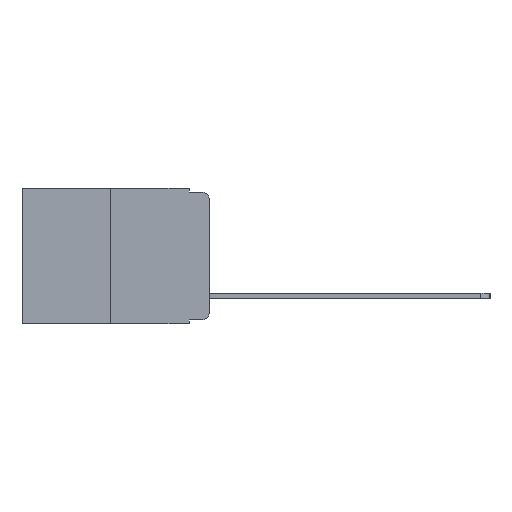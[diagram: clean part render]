
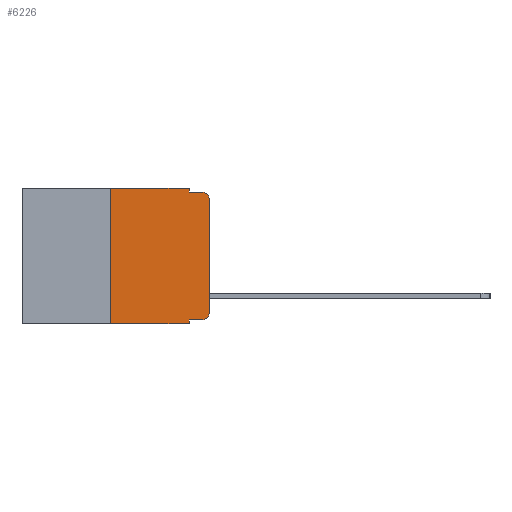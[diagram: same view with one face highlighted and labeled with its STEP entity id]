
A CAD part, left-side view. The second image highlights one B-rep face of the part: STEP entity #6226.
In plain terms, the highlighted planar face has unit normal (-1, 0, 0).
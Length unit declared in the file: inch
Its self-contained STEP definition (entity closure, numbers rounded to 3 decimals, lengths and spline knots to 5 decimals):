
#80 = DIRECTION ( 'NONE',  ( 0., -1., 0. ) ) ;
#190 = CARTESIAN_POINT ( 'NONE',  ( 0., 0.473, 0. ) ) ;
#302 = VERTEX_POINT ( 'NONE', #14236 ) ;
#464 = LINE ( 'NONE', #7982, #3529 ) ;
#611 = VERTEX_POINT ( 'NONE', #10614 ) ;
#622 = ORIENTED_EDGE ( 'NONE', *, *, #9368, .F. ) ;
#929 = EDGE_CURVE ( 'NONE', #302, #2626, #15216, .T. ) ;
#1022 = DIRECTION ( 'NONE',  ( -1., 0., 0. ) ) ;
#1023 = DIRECTION ( 'NONE',  ( 0., 0., -1. ) ) ;
#1599 = DIRECTION ( 'NONE',  ( 1., 0., 0. ) ) ;
#1757 = EDGE_CURVE ( 'NONE', #7967, #7173, #464, .T. ) ;
#2019 = CARTESIAN_POINT ( 'NONE',  ( 0., 0.25, 0. ) ) ;
#2097 = VECTOR ( 'NONE', #10262, 39.37008 ) ;
#2626 = VERTEX_POINT ( 'NONE', #9595 ) ;
#2838 = PLANE ( 'NONE',  #9090 ) ;
#2847 = ORIENTED_EDGE ( 'NONE', *, *, #3936, .F. ) ;
#2858 = LINE ( 'NONE', #5931, #15145 ) ;
#2879 = EDGE_CURVE ( 'NONE', #7972, #7967, #13456, .T. ) ;
#2944 = AXIS2_PLACEMENT_3D ( 'NONE', #8415, #1022, #9590 ) ;
#2963 = CARTESIAN_POINT ( 'NONE',  ( 0., 0.051, -0.333 ) ) ;
#2991 = CARTESIAN_POINT ( 'NONE',  ( 0., 0.051, -0.01 ) ) ;
#3304 = LINE ( 'NONE', #12311, #9719 ) ;
#3348 = EDGE_CURVE ( 'NONE', #302, #7972, #14471, .T. ) ;
#3385 = DIRECTION ( 'NONE',  ( -1., 0., 0. ) ) ;
#3418 = VECTOR ( 'NONE', #11249, 39.37008 ) ;
#3433 = CARTESIAN_POINT ( 'NONE',  ( 0., 0.02, -0.313 ) ) ;
#3529 = VECTOR ( 'NONE', #7605, 39.37008 ) ;
#3860 = DIRECTION ( 'NONE',  ( 0., -1., 0. ) ) ;
#3936 = EDGE_CURVE ( 'NONE', #6703, #5242, #5346, .T. ) ;
#4079 = VERTEX_POINT ( 'NONE', #15655 ) ;
#4411 = AXIS2_PLACEMENT_3D ( 'NONE', #3433, #3385, #12573 ) ;
#4715 = EDGE_CURVE ( 'NONE', #4079, #2626, #2858, .T. ) ;
#5242 = VERTEX_POINT ( 'NONE', #14704 ) ;
#5346 = LINE ( 'NONE', #2991, #2097 ) ;
#5667 = CARTESIAN_POINT ( 'NONE',  ( 0., 0.051, -0.01 ) ) ;
#5921 = CARTESIAN_POINT ( 'NONE',  ( 0., 0.051, 0. ) ) ;
#5931 = CARTESIAN_POINT ( 'NONE',  ( 0., 0.473, -0.343 ) ) ;
#6226 = ADVANCED_FACE ( 'NONE', ( #8186 ), #2838, .F. ) ;
#6314 = ORIENTED_EDGE ( 'NONE', *, *, #1757, .T. ) ;
#6367 = EDGE_LOOP ( 'NONE', ( #6314, #9865, #2847, #622, #13597, #11990, #10676, #11414, #14465, #12910 ) ) ;
#6418 = CARTESIAN_POINT ( 'NONE',  ( 0., 0.25, 0. ) ) ;
#6506 = DIRECTION ( 'NONE',  ( 0., 0., -1. ) ) ;
#6703 = VERTEX_POINT ( 'NONE', #5667 ) ;
#7005 = EDGE_CURVE ( 'NONE', #4079, #8303, #9039, .T. ) ;
#7173 = VERTEX_POINT ( 'NONE', #8062 ) ;
#7464 = EDGE_CURVE ( 'NONE', #8303, #611, #3304, .T. ) ;
#7605 = DIRECTION ( 'NONE',  ( 0., 0., 1. ) ) ;
#7967 = VERTEX_POINT ( 'NONE', #12347 ) ;
#7972 = VERTEX_POINT ( 'NONE', #14587 ) ;
#7982 = CARTESIAN_POINT ( 'NONE',  ( 0., 0., 0. ) ) ;
#8062 = CARTESIAN_POINT ( 'NONE',  ( 0., 0., -0.03 ) ) ;
#8186 = FACE_OUTER_BOUND ( 'NONE', #6367, .T. ) ;
#8303 = VERTEX_POINT ( 'NONE', #2019 ) ;
#8415 = CARTESIAN_POINT ( 'NONE',  ( 0., 0.02, -0.03 ) ) ;
#8793 = EDGE_CURVE ( 'NONE', #7173, #5242, #11758, .T. ) ;
#8812 = CARTESIAN_POINT ( 'NONE',  ( 0., 0.051, 0. ) ) ;
#9012 = VECTOR ( 'NONE', #1023, 39.37008 ) ;
#9039 = LINE ( 'NONE', #6418, #14891 ) ;
#9090 = AXIS2_PLACEMENT_3D ( 'NONE', #190, #1599, #6506 ) ;
#9368 = EDGE_CURVE ( 'NONE', #611, #6703, #13378, .T. ) ;
#9590 = DIRECTION ( 'NONE',  ( 0., 0., -1. ) ) ;
#9595 = CARTESIAN_POINT ( 'NONE',  ( 0., 0.051, -0.343 ) ) ;
#9719 = VECTOR ( 'NONE', #3860, 39.37008 ) ;
#9865 = ORIENTED_EDGE ( 'NONE', *, *, #8793, .T. ) ;
#10262 = DIRECTION ( 'NONE',  ( 0., -1., 0. ) ) ;
#10614 = CARTESIAN_POINT ( 'NONE',  ( 0., 0.051, 0. ) ) ;
#10676 = ORIENTED_EDGE ( 'NONE', *, *, #4715, .T. ) ;
#11249 = DIRECTION ( 'NONE',  ( 0., 0., -1. ) ) ;
#11414 = ORIENTED_EDGE ( 'NONE', *, *, #929, .F. ) ;
#11421 = VECTOR ( 'NONE', #80, 39.37008 ) ;
#11758 = CIRCLE ( 'NONE', #2944, 0.02 ) ;
#11990 = ORIENTED_EDGE ( 'NONE', *, *, #7005, .F. ) ;
#12311 = CARTESIAN_POINT ( 'NONE',  ( 0., 0.473, 0. ) ) ;
#12347 = CARTESIAN_POINT ( 'NONE',  ( 0., 0., -0.313 ) ) ;
#12573 = DIRECTION ( 'NONE',  ( 0., 0., -1. ) ) ;
#12849 = DIRECTION ( 'NONE',  ( 0., -1., 0. ) ) ;
#12910 = ORIENTED_EDGE ( 'NONE', *, *, #2879, .T. ) ;
#13378 = LINE ( 'NONE', #8812, #3418 ) ;
#13456 = CIRCLE ( 'NONE', #4411, 0.02 ) ;
#13559 = DIRECTION ( 'NONE',  ( 0., 0., 1. ) ) ;
#13597 = ORIENTED_EDGE ( 'NONE', *, *, #7464, .F. ) ;
#14236 = CARTESIAN_POINT ( 'NONE',  ( 0., 0.051, -0.333 ) ) ;
#14465 = ORIENTED_EDGE ( 'NONE', *, *, #3348, .T. ) ;
#14471 = LINE ( 'NONE', #2963, #11421 ) ;
#14587 = CARTESIAN_POINT ( 'NONE',  ( 0., 0.02, -0.333 ) ) ;
#14704 = CARTESIAN_POINT ( 'NONE',  ( 0., 0.02, -0.01 ) ) ;
#14891 = VECTOR ( 'NONE', #13559, 39.37008 ) ;
#15145 = VECTOR ( 'NONE', #12849, 39.37008 ) ;
#15216 = LINE ( 'NONE', #5921, #9012 ) ;
#15655 = CARTESIAN_POINT ( 'NONE',  ( 0., 0.25, -0.343 ) ) ;
